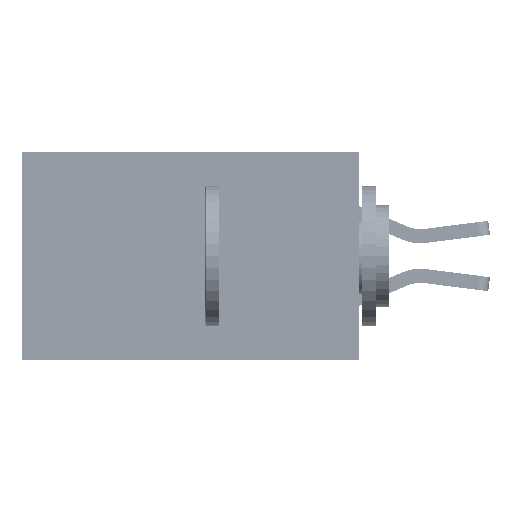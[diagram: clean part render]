
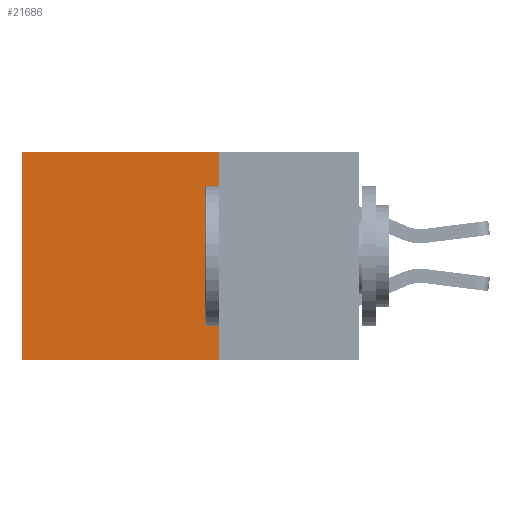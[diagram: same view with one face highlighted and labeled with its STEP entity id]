
A CAD part, left-side view. The second image highlights one B-rep face of the part: STEP entity #21686.
In plain terms, the highlighted planar face has unit normal (-1, 0, 0).
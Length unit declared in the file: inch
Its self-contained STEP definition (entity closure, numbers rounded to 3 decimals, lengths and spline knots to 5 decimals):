
#998 = VECTOR ( 'NONE', #37863, 39.37008 ) ;
#1567 = EDGE_CURVE ( 'NONE', #16767, #9041, #43409, .T. ) ;
#2119 = LINE ( 'NONE', #2452, #998 ) ;
#2321 = ORIENTED_EDGE ( 'NONE', *, *, #28262, .F. ) ;
#2452 = CARTESIAN_POINT ( 'NONE',  ( 0.2875, 0.25, 0. ) ) ;
#3443 = CARTESIAN_POINT ( 'NONE',  ( 0.2875, 0.25, -0.37 ) ) ;
#4986 = EDGE_CURVE ( 'NONE', #41404, #13457, #36340, .T. ) ;
#6763 = ORIENTED_EDGE ( 'NONE', *, *, #4986, .F. ) ;
#8847 = DIRECTION ( 'NONE',  ( 0., 1., 0. ) ) ;
#9041 = VERTEX_POINT ( 'NONE', #42168 ) ;
#12619 = DIRECTION ( 'NONE',  ( 1., 0., 0. ) ) ;
#12720 = CARTESIAN_POINT ( 'NONE',  ( 0.2875, 0.6, 0. ) ) ;
#13457 = VERTEX_POINT ( 'NONE', #3443 ) ;
#13857 = EDGE_CURVE ( 'NONE', #41404, #16767, #2119, .T. ) ;
#16317 = AXIS2_PLACEMENT_3D ( 'NONE', #43963, #12619, #37285 ) ;
#16422 = VECTOR ( 'NONE', #8847, 39.37008 ) ;
#16767 = VERTEX_POINT ( 'NONE', #40122 ) ;
#17591 = VECTOR ( 'NONE', #39407, 39.37008 ) ;
#18338 = CARTESIAN_POINT ( 'NONE',  ( 0.2875, 0.25, 0. ) ) ;
#21686 = ADVANCED_FACE ( 'NONE', ( #26927 ), #33838, .F. ) ;
#21717 = ORIENTED_EDGE ( 'NONE', *, *, #1567, .T. ) ;
#26927 = FACE_OUTER_BOUND ( 'NONE', #39667, .T. ) ;
#28262 = EDGE_CURVE ( 'NONE', #13457, #9041, #35232, .T. ) ;
#29957 = CARTESIAN_POINT ( 'NONE',  ( 0.2875, 0.25, -0.37 ) ) ;
#33838 = PLANE ( 'NONE',  #16317 ) ;
#34214 = ORIENTED_EDGE ( 'NONE', *, *, #13857, .T. ) ;
#34217 = VECTOR ( 'NONE', #44358, 39.37008 ) ;
#35232 = LINE ( 'NONE', #29957, #16422 ) ;
#36340 = LINE ( 'NONE', #18338, #17591 ) ;
#37285 = DIRECTION ( 'NONE',  ( 0., 0., -1. ) ) ;
#37863 = DIRECTION ( 'NONE',  ( 0., 1., 0. ) ) ;
#39407 = DIRECTION ( 'NONE',  ( 0., 0., -1. ) ) ;
#39667 = EDGE_LOOP ( 'NONE', ( #21717, #2321, #6763, #34214 ) ) ;
#40122 = CARTESIAN_POINT ( 'NONE',  ( 0.2875, 0.6, 0. ) ) ;
#41404 = VERTEX_POINT ( 'NONE', #43721 ) ;
#42168 = CARTESIAN_POINT ( 'NONE',  ( 0.2875, 0.6, -0.37 ) ) ;
#43409 = LINE ( 'NONE', #12720, #34217 ) ;
#43721 = CARTESIAN_POINT ( 'NONE',  ( 0.2875, 0.25, 0. ) ) ;
#43963 = CARTESIAN_POINT ( 'NONE',  ( 0.2875, 0.25, 0. ) ) ;
#44358 = DIRECTION ( 'NONE',  ( 0., 0., -1. ) ) ;
